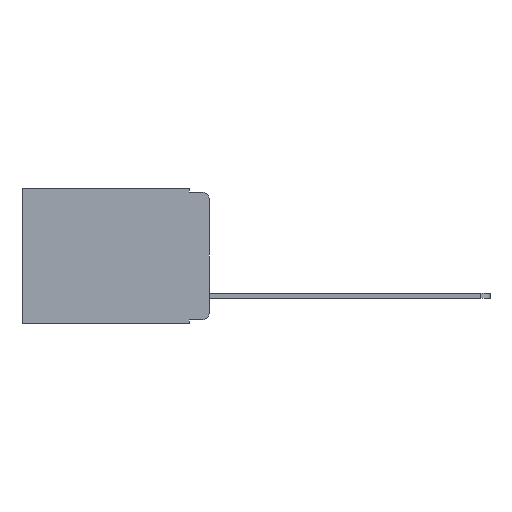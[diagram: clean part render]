
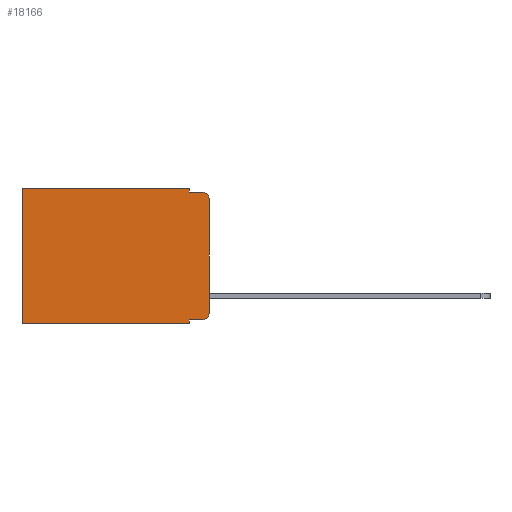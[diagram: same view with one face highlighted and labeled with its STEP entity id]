
A CAD part, left-side view. The second image highlights one B-rep face of the part: STEP entity #18166.
In plain terms, the highlighted planar face has unit normal (-1, 0, 0).
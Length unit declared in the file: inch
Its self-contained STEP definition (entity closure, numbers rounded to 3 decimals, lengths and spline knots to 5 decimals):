
#297 = DIRECTION ( 'NONE',  ( 0., 0., -1. ) ) ;
#370 = DIRECTION ( 'NONE',  ( 0., 0., -1. ) ) ;
#535 = CARTESIAN_POINT ( 'NONE',  ( 0.298, 0.051, 0. ) ) ;
#815 = LINE ( 'NONE', #1939, #8663 ) ;
#1748 = VERTEX_POINT ( 'NONE', #6173 ) ;
#1907 = CIRCLE ( 'NONE', #11445, 0.02 ) ;
#1939 = CARTESIAN_POINT ( 'NONE',  ( 0.298, 0.051, 0. ) ) ;
#1982 = EDGE_CURVE ( 'NONE', #5964, #19530, #1907, .T. ) ;
#2622 = LINE ( 'NONE', #16253, #18550 ) ;
#2710 = ORIENTED_EDGE ( 'NONE', *, *, #19913, .F. ) ;
#2747 = DIRECTION ( 'NONE',  ( 0., 0., -1. ) ) ;
#2882 = VERTEX_POINT ( 'NONE', #12112 ) ;
#3623 = VERTEX_POINT ( 'NONE', #6122 ) ;
#3875 = CARTESIAN_POINT ( 'NONE',  ( 0.298, 0.051, -0.01 ) ) ;
#4095 = DIRECTION ( 'NONE',  ( 0., 1., 0. ) ) ;
#4107 = LINE ( 'NONE', #5334, #12394 ) ;
#4255 = CARTESIAN_POINT ( 'NONE',  ( 0.298, 0., -0.03 ) ) ;
#4593 = LINE ( 'NONE', #7330, #12869 ) ;
#4610 = EDGE_CURVE ( 'NONE', #3623, #13989, #4107, .T. ) ;
#4903 = ORIENTED_EDGE ( 'NONE', *, *, #16876, .F. ) ;
#5123 = EDGE_CURVE ( 'NONE', #5964, #2882, #2622, .T. ) ;
#5334 = CARTESIAN_POINT ( 'NONE',  ( 0.298, 0., 0. ) ) ;
#5854 = LINE ( 'NONE', #11660, #17636 ) ;
#5904 = ORIENTED_EDGE ( 'NONE', *, *, #15876, .T. ) ;
#5964 = VERTEX_POINT ( 'NONE', #4255 ) ;
#6122 = CARTESIAN_POINT ( 'NONE',  ( 0.298, 0.051, 0. ) ) ;
#6173 = CARTESIAN_POINT ( 'NONE',  ( 0.298, 0.473, -0.343 ) ) ;
#6400 = DIRECTION ( 'NONE',  ( 0., 0., -1. ) ) ;
#6419 = FACE_OUTER_BOUND ( 'NONE', #19874, .T. ) ;
#6692 = AXIS2_PLACEMENT_3D ( 'NONE', #12010, #7373, #18108 ) ;
#6791 = DIRECTION ( 'NONE',  ( 0., 1., 0. ) ) ;
#6912 = LINE ( 'NONE', #15032, #14678 ) ;
#6970 = LINE ( 'NONE', #535, #7444 ) ;
#6982 = VERTEX_POINT ( 'NONE', #3875 ) ;
#7152 = ORIENTED_EDGE ( 'NONE', *, *, #9672, .T. ) ;
#7330 = CARTESIAN_POINT ( 'NONE',  ( 0.298, 0.051, -0.333 ) ) ;
#7373 = DIRECTION ( 'NONE',  ( 1., 0., 0. ) ) ;
#7444 = VECTOR ( 'NONE', #16062, 39.37008 ) ;
#8081 = ORIENTED_EDGE ( 'NONE', *, *, #1982, .T. ) ;
#8663 = VECTOR ( 'NONE', #370, 39.37008 ) ;
#9313 = ORIENTED_EDGE ( 'NONE', *, *, #4610, .T. ) ;
#9537 = VERTEX_POINT ( 'NONE', #20048 ) ;
#9672 = EDGE_CURVE ( 'NONE', #9537, #2882, #19069, .T. ) ;
#9696 = DIRECTION ( 'NONE',  ( -1., 0., 0. ) ) ;
#10016 = ORIENTED_EDGE ( 'NONE', *, *, #5123, .F. ) ;
#10017 = VECTOR ( 'NONE', #2747, 39.37008 ) ;
#10246 = ORIENTED_EDGE ( 'NONE', *, *, #11787, .T. ) ;
#11004 = VERTEX_POINT ( 'NONE', #18959 ) ;
#11185 = VERTEX_POINT ( 'NONE', #19334 ) ;
#11445 = AXIS2_PLACEMENT_3D ( 'NONE', #16108, #18298, #6400 ) ;
#11660 = CARTESIAN_POINT ( 'NONE',  ( 0.298, 0.051, -0.01 ) ) ;
#11727 = DIRECTION ( 'NONE',  ( 0., -1., 0. ) ) ;
#11787 = EDGE_CURVE ( 'NONE', #11185, #9537, #4593, .T. ) ;
#11971 = DIRECTION ( 'NONE',  ( 0., -1., 0. ) ) ;
#12010 = CARTESIAN_POINT ( 'NONE',  ( 0.298, 0., 0. ) ) ;
#12092 = CARTESIAN_POINT ( 'NONE',  ( 0.298, 0.473, 0. ) ) ;
#12112 = CARTESIAN_POINT ( 'NONE',  ( 0.298, 0., -0.313 ) ) ;
#12394 = VECTOR ( 'NONE', #6791, 39.37008 ) ;
#12415 = DIRECTION ( 'NONE',  ( 0., 0., -1. ) ) ;
#12817 = AXIS2_PLACEMENT_3D ( 'NONE', #18869, #9696, #297 ) ;
#12869 = VECTOR ( 'NONE', #11971, 39.37008 ) ;
#13841 = CARTESIAN_POINT ( 'NONE',  ( 0.298, 0.02, -0.01 ) ) ;
#13867 = EDGE_CURVE ( 'NONE', #11185, #11004, #815, .T. ) ;
#13989 = VERTEX_POINT ( 'NONE', #19183 ) ;
#14176 = LINE ( 'NONE', #12092, #10017 ) ;
#14678 = VECTOR ( 'NONE', #4095, 39.37008 ) ;
#15032 = CARTESIAN_POINT ( 'NONE',  ( 0.298, 0., -0.343 ) ) ;
#15876 = EDGE_CURVE ( 'NONE', #13989, #1748, #14176, .T. ) ;
#16062 = DIRECTION ( 'NONE',  ( 0., 0., -1. ) ) ;
#16108 = CARTESIAN_POINT ( 'NONE',  ( 0.298, 0.02, -0.03 ) ) ;
#16253 = CARTESIAN_POINT ( 'NONE',  ( 0.298, 0., 0. ) ) ;
#16593 = PLANE ( 'NONE',  #6692 ) ;
#16876 = EDGE_CURVE ( 'NONE', #3623, #6982, #6970, .T. ) ;
#17225 = ORIENTED_EDGE ( 'NONE', *, *, #18141, .F. ) ;
#17636 = VECTOR ( 'NONE', #11727, 39.37008 ) ;
#18108 = DIRECTION ( 'NONE',  ( 0., 0., -1. ) ) ;
#18141 = EDGE_CURVE ( 'NONE', #11004, #1748, #6912, .T. ) ;
#18166 = ADVANCED_FACE ( 'NONE', ( #6419 ), #16593, .F. ) ;
#18298 = DIRECTION ( 'NONE',  ( -1., 0., 0. ) ) ;
#18550 = VECTOR ( 'NONE', #12415, 39.37008 ) ;
#18639 = ORIENTED_EDGE ( 'NONE', *, *, #13867, .F. ) ;
#18869 = CARTESIAN_POINT ( 'NONE',  ( 0.298, 0.02, -0.313 ) ) ;
#18959 = CARTESIAN_POINT ( 'NONE',  ( 0.298, 0.051, -0.343 ) ) ;
#19069 = CIRCLE ( 'NONE', #12817, 0.02 ) ;
#19183 = CARTESIAN_POINT ( 'NONE',  ( 0.298, 0.473, 0. ) ) ;
#19334 = CARTESIAN_POINT ( 'NONE',  ( 0.298, 0.051, -0.333 ) ) ;
#19530 = VERTEX_POINT ( 'NONE', #13841 ) ;
#19874 = EDGE_LOOP ( 'NONE', ( #10016, #8081, #2710, #4903, #9313, #5904, #17225, #18639, #10246, #7152 ) ) ;
#19913 = EDGE_CURVE ( 'NONE', #6982, #19530, #5854, .T. ) ;
#20048 = CARTESIAN_POINT ( 'NONE',  ( 0.298, 0.02, -0.333 ) ) ;
